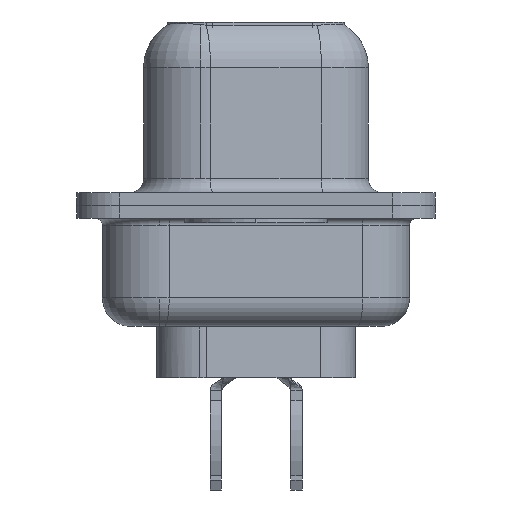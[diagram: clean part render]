
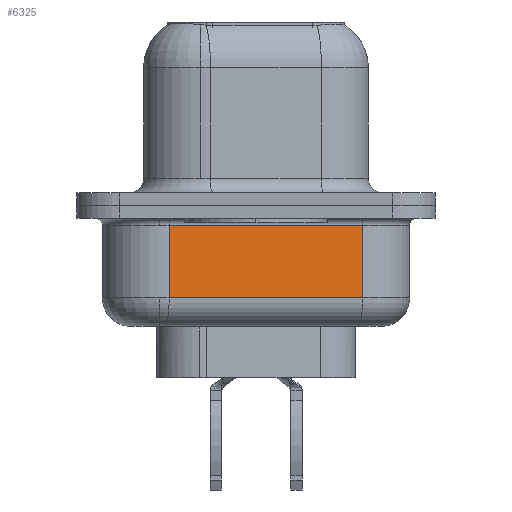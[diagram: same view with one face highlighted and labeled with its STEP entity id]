
A CAD part, left-side view. The second image highlights one B-rep face of the part: STEP entity #6325.
In plain terms, the highlighted planar face has unit normal (-0.985, -0.174, 0).
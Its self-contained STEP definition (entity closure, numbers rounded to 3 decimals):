
#196 = DIRECTION ( 'NONE',  ( 0.985, 0.174, 0. ) ) ;
#572 = VERTEX_POINT ( 'NONE', #9321 ) ;
#657 = ORIENTED_EDGE ( 'NONE', *, *, #12259, .T. ) ;
#714 = EDGE_CURVE ( 'NONE', #572, #851, #12282, .T. ) ;
#806 = EDGE_CURVE ( 'NONE', #8372, #851, #12819, .T. ) ;
#851 = VERTEX_POINT ( 'NONE', #11628 ) ;
#1528 = DIRECTION ( 'NONE',  ( -0.174, 0.985, 0. ) ) ;
#1665 = VECTOR ( 'NONE', #1528, 1000. ) ;
#2980 = EDGE_CURVE ( 'NONE', #10125, #8372, #17236, .T. ) ;
#3854 = LINE ( 'NONE', #9434, #4174 ) ;
#4174 = VECTOR ( 'NONE', #14770, 1000. ) ;
#4192 = CARTESIAN_POINT ( 'NONE',  ( 2.875, 3.053, -4.25 ) ) ;
#5388 = ORIENTED_EDGE ( 'NONE', *, *, #806, .T. ) ;
#5481 = ORIENTED_EDGE ( 'NONE', *, *, #2980, .T. ) ;
#5773 = ORIENTED_EDGE ( 'NONE', *, *, #714, .F. ) ;
#6325 = ADVANCED_FACE ( 'NONE', ( #7172 ), #8992, .F. ) ;
#7172 = FACE_OUTER_BOUND ( 'NONE', #9727, .T. ) ;
#7646 = DIRECTION ( 'NONE',  ( 0., 0., 1. ) ) ;
#8372 = VERTEX_POINT ( 'NONE', #11634 ) ;
#8631 = DIRECTION ( 'NONE',  ( -0.174, 0.985, 0. ) ) ;
#8992 = PLANE ( 'NONE',  #17103 ) ;
#9321 = CARTESIAN_POINT ( 'NONE',  ( 2.875, 3.053, -3.25 ) ) ;
#9434 = CARTESIAN_POINT ( 'NONE',  ( 2.875, 3.053, -3.25 ) ) ;
#9571 = VECTOR ( 'NONE', #14019, 1000. ) ;
#9727 = EDGE_LOOP ( 'NONE', ( #5773, #657, #5481, #5388 ) ) ;
#10125 = VERTEX_POINT ( 'NONE', #13346 ) ;
#11121 = VECTOR ( 'NONE', #7646, 1000. ) ;
#11628 = CARTESIAN_POINT ( 'NONE',  ( 2.875, 3.053, -0.7 ) ) ;
#11634 = CARTESIAN_POINT ( 'NONE',  ( 4.074, -3.747, -0.7 ) ) ;
#12259 = EDGE_CURVE ( 'NONE', #572, #10125, #3854, .T. ) ;
#12282 = LINE ( 'NONE', #4192, #9571 ) ;
#12774 = CARTESIAN_POINT ( 'NONE',  ( 2.875, 3.053, -4.25 ) ) ;
#12819 = LINE ( 'NONE', #15771, #1665 ) ;
#13346 = CARTESIAN_POINT ( 'NONE',  ( 4.074, -3.747, -3.25 ) ) ;
#14019 = DIRECTION ( 'NONE',  ( 0., 0., 1. ) ) ;
#14452 = CARTESIAN_POINT ( 'NONE',  ( 4.074, -3.747, -4.25 ) ) ;
#14770 = DIRECTION ( 'NONE',  ( 0.174, -0.985, 0. ) ) ;
#15771 = CARTESIAN_POINT ( 'NONE',  ( 2.875, 3.053, -0.7 ) ) ;
#17103 = AXIS2_PLACEMENT_3D ( 'NONE', #12774, #196, #8631 ) ;
#17236 = LINE ( 'NONE', #14452, #11121 ) ;
